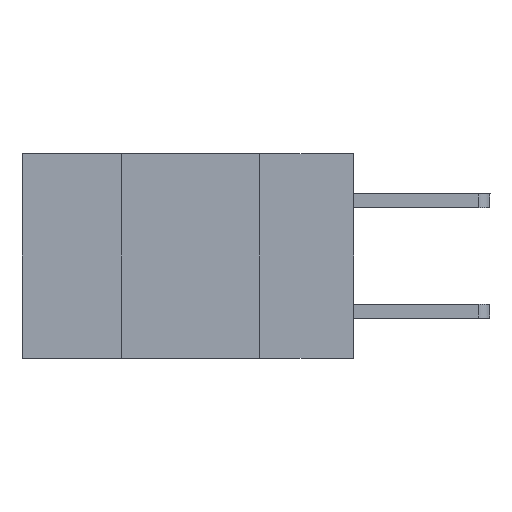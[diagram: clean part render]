
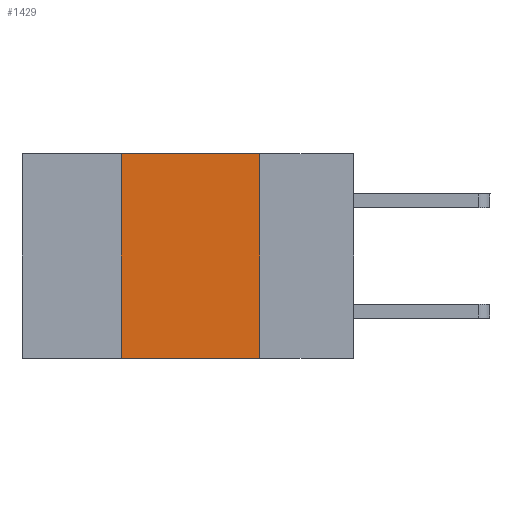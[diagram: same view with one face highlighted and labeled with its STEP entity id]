
A CAD part, left-side view. The second image highlights one B-rep face of the part: STEP entity #1429.
In plain terms, the highlighted planar face has unit normal (-1, 0, 0).
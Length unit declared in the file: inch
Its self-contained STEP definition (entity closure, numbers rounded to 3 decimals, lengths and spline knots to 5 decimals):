
#330 = CARTESIAN_POINT ( 'NONE',  ( 0., 0.6, 0. ) ) ;
#545 = EDGE_CURVE ( 'NONE', #10406, #4962, #8013, .T. ) ;
#694 = EDGE_CURVE ( 'NONE', #3884, #10406, #4857, .T. ) ;
#1318 = DIRECTION ( 'NONE',  ( 0., 0., -1. ) ) ;
#1349 = CARTESIAN_POINT ( 'NONE',  ( 0., 0.17, 0. ) ) ;
#1429 = ADVANCED_FACE ( 'NONE', ( #9383 ), #3395, .F. ) ;
#1440 = ORIENTED_EDGE ( 'NONE', *, *, #694, .F. ) ;
#1464 = EDGE_LOOP ( 'NONE', ( #3220, #1440, #3662, #6193 ) ) ;
#1736 = EDGE_CURVE ( 'NONE', #4523, #4962, #5115, .T. ) ;
#1795 = CARTESIAN_POINT ( 'NONE',  ( 0., 0.17, 0. ) ) ;
#1925 = DIRECTION ( 'NONE',  ( 0., 0., 1. ) ) ;
#2906 = CARTESIAN_POINT ( 'NONE',  ( 0., 0.6, 0. ) ) ;
#2991 = AXIS2_PLACEMENT_3D ( 'NONE', #2906, #10697, #1318 ) ;
#3006 = CARTESIAN_POINT ( 'NONE',  ( 0., 0.6, -0.37 ) ) ;
#3220 = ORIENTED_EDGE ( 'NONE', *, *, #545, .F. ) ;
#3395 = PLANE ( 'NONE',  #2991 ) ;
#3662 = ORIENTED_EDGE ( 'NONE', *, *, #8794, .F. ) ;
#3884 = VERTEX_POINT ( 'NONE', #3926 ) ;
#3926 = CARTESIAN_POINT ( 'NONE',  ( 0., 0.42, 0. ) ) ;
#4523 = VERTEX_POINT ( 'NONE', #8980 ) ;
#4581 = VECTOR ( 'NONE', #8165, 39.37008 ) ;
#4857 = LINE ( 'NONE', #330, #4581 ) ;
#4962 = VERTEX_POINT ( 'NONE', #5565 ) ;
#5115 = LINE ( 'NONE', #3006, #10230 ) ;
#5565 = CARTESIAN_POINT ( 'NONE',  ( 0., 0.17, -0.37 ) ) ;
#6193 = ORIENTED_EDGE ( 'NONE', *, *, #1736, .T. ) ;
#6571 = LINE ( 'NONE', #10809, #8908 ) ;
#7034 = VECTOR ( 'NONE', #7969, 39.37008 ) ;
#7969 = DIRECTION ( 'NONE',  ( 0., 0., -1. ) ) ;
#8013 = LINE ( 'NONE', #1795, #7034 ) ;
#8165 = DIRECTION ( 'NONE',  ( 0., -1., 0. ) ) ;
#8794 = EDGE_CURVE ( 'NONE', #4523, #3884, #6571, .T. ) ;
#8908 = VECTOR ( 'NONE', #1925, 39.37008 ) ;
#8980 = CARTESIAN_POINT ( 'NONE',  ( 0., 0.42, -0.37 ) ) ;
#9383 = FACE_OUTER_BOUND ( 'NONE', #1464, .T. ) ;
#10094 = DIRECTION ( 'NONE',  ( 0., -1., 0. ) ) ;
#10230 = VECTOR ( 'NONE', #10094, 39.37008 ) ;
#10406 = VERTEX_POINT ( 'NONE', #1349 ) ;
#10697 = DIRECTION ( 'NONE',  ( 1., 0., 0. ) ) ;
#10809 = CARTESIAN_POINT ( 'NONE',  ( 0., 0.42, 0. ) ) ;
